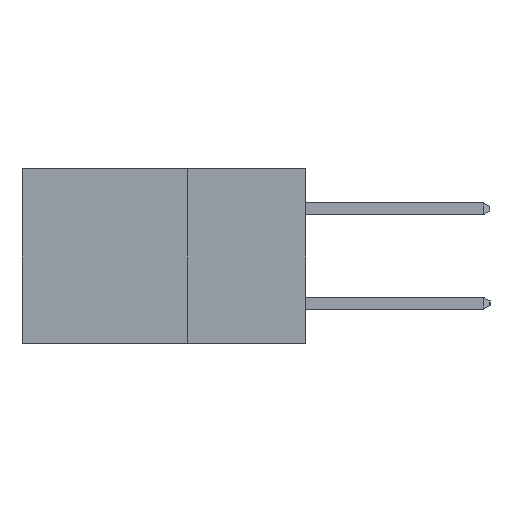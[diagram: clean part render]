
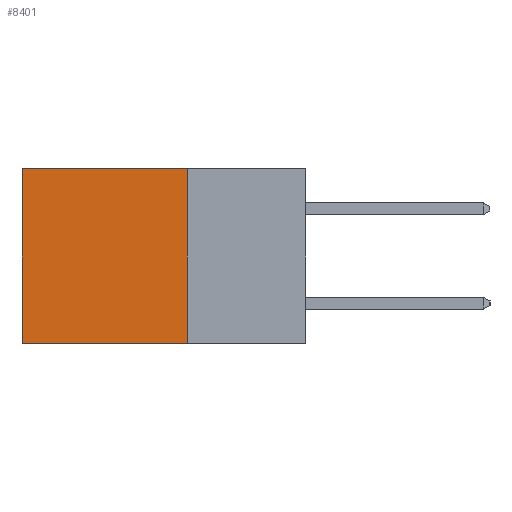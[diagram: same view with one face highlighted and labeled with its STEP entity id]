
A CAD part, left-side view. The second image highlights one B-rep face of the part: STEP entity #8401.
In plain terms, the highlighted planar face has unit normal (-1, 0, 0).
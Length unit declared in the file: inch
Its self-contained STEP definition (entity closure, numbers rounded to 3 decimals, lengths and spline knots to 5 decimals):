
#415 = EDGE_CURVE ( 'NONE', #8060, #15153, #12079, .T. ) ;
#898 = VECTOR ( 'NONE', #7834, 39.37008 ) ;
#1171 = PLANE ( 'NONE',  #10599 ) ;
#2166 = VECTOR ( 'NONE', #12252, 39.37008 ) ;
#2524 = ORIENTED_EDGE ( 'NONE', *, *, #11968, .T. ) ;
#2638 = CARTESIAN_POINT ( 'NONE',  ( 0.2615, 0.25, -0.37 ) ) ;
#2697 = VECTOR ( 'NONE', #7820, 39.37008 ) ;
#2728 = DIRECTION ( 'NONE',  ( 0., 0., -1. ) ) ;
#3427 = VERTEX_POINT ( 'NONE', #8233 ) ;
#4060 = EDGE_CURVE ( 'NONE', #8060, #3427, #9322, .T. ) ;
#5316 = ORIENTED_EDGE ( 'NONE', *, *, #415, .F. ) ;
#6785 = ORIENTED_EDGE ( 'NONE', *, *, #4060, .T. ) ;
#6915 = CARTESIAN_POINT ( 'NONE',  ( 0.2615, 0.25, -0.37 ) ) ;
#7250 = VECTOR ( 'NONE', #14121, 39.37008 ) ;
#7820 = DIRECTION ( 'NONE',  ( 0., 0., -1. ) ) ;
#7834 = DIRECTION ( 'NONE',  ( 0., 0., -1. ) ) ;
#7984 = CARTESIAN_POINT ( 'NONE',  ( 0.2615, 0.6, -0.37 ) ) ;
#8036 = CARTESIAN_POINT ( 'NONE',  ( 0.2615, 0.25, -0.37 ) ) ;
#8052 = FACE_OUTER_BOUND ( 'NONE', #8264, .T. ) ;
#8060 = VERTEX_POINT ( 'NONE', #9118 ) ;
#8233 = CARTESIAN_POINT ( 'NONE',  ( 0.2615, 0.6, 0. ) ) ;
#8264 = EDGE_LOOP ( 'NONE', ( #2524, #15648, #5316, #6785 ) ) ;
#8401 = ADVANCED_FACE ( 'NONE', ( #8052 ), #1171, .F. ) ;
#9118 = CARTESIAN_POINT ( 'NONE',  ( 0.2615, 0.25, 0. ) ) ;
#9179 = LINE ( 'NONE', #2638, #2166 ) ;
#9322 = LINE ( 'NONE', #14890, #7250 ) ;
#9517 = CARTESIAN_POINT ( 'NONE',  ( 0.2615, 0.25, -0.37 ) ) ;
#10054 = LINE ( 'NONE', #15847, #2697 ) ;
#10599 = AXIS2_PLACEMENT_3D ( 'NONE', #6915, #10996, #2728 ) ;
#10996 = DIRECTION ( 'NONE',  ( 1., 0., 0. ) ) ;
#11968 = EDGE_CURVE ( 'NONE', #3427, #15719, #10054, .T. ) ;
#12079 = LINE ( 'NONE', #8036, #898 ) ;
#12252 = DIRECTION ( 'NONE',  ( 0., 1., 0. ) ) ;
#12910 = EDGE_CURVE ( 'NONE', #15153, #15719, #9179, .T. ) ;
#14121 = DIRECTION ( 'NONE',  ( 0., 1., 0. ) ) ;
#14890 = CARTESIAN_POINT ( 'NONE',  ( 0.2615, 0.25, 0. ) ) ;
#15153 = VERTEX_POINT ( 'NONE', #9517 ) ;
#15648 = ORIENTED_EDGE ( 'NONE', *, *, #12910, .F. ) ;
#15719 = VERTEX_POINT ( 'NONE', #7984 ) ;
#15847 = CARTESIAN_POINT ( 'NONE',  ( 0.2615, 0.6, -0.37 ) ) ;
